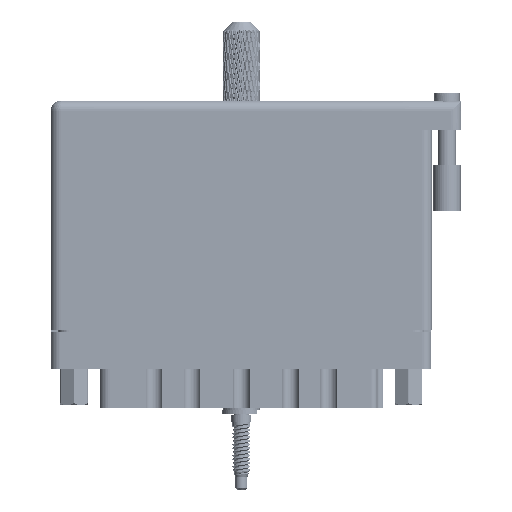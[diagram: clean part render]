
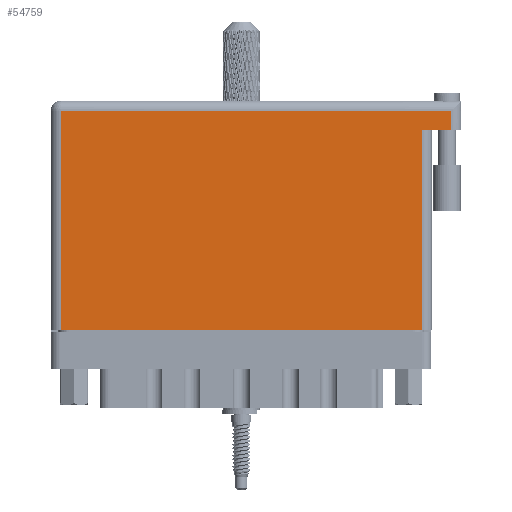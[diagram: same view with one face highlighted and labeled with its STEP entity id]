
A CAD part, front view. The second image highlights one B-rep face of the part: STEP entity #54759.
In plain terms, the highlighted face is planar.
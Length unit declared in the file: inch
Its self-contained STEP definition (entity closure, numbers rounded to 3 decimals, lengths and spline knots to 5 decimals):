
#682 = VERTEX_POINT ( 'NONE', #94941 ) ;
#1502 = VECTOR ( 'NONE', #6247, 39.37008 ) ;
#2481 = ORIENTED_EDGE ( 'NONE', *, *, #22006, .T. ) ;
#2527 = LINE ( 'NONE', #58421, #116686 ) ;
#3519 = EDGE_CURVE ( 'NONE', #682, #115316, #29239, .T. ) ;
#5059 = CARTESIAN_POINT ( 'NONE',  ( 0.07, 1.496, 0. ) ) ;
#6247 = DIRECTION ( 'NONE',  ( 1., 0., 0. ) ) ;
#7008 = ORIENTED_EDGE ( 'NONE', *, *, #46741, .T. ) ;
#7679 = VECTOR ( 'NONE', #100593, 39.37008 ) ;
#9228 = CARTESIAN_POINT ( 'NONE',  ( 2.8, 1.369, 0. ) ) ;
#10385 = VECTOR ( 'NONE', #109927, 39.37008 ) ;
#12273 = LINE ( 'NONE', #121031, #61718 ) ;
#16491 = VECTOR ( 'NONE', #57573, 39.37008 ) ;
#22006 = EDGE_CURVE ( 'NONE', #51543, #46863, #2527, .T. ) ;
#22716 = VERTEX_POINT ( 'NONE', #110933 ) ;
#28659 = CARTESIAN_POINT ( 'NONE',  ( 2.53, 1.369, 0. ) ) ;
#29239 = LINE ( 'NONE', #111358, #7679 ) ;
#31530 = CARTESIAN_POINT ( 'NONE',  ( 2.73, 1.566, 0. ) ) ;
#33336 = CARTESIAN_POINT ( 'NONE',  ( 0.07, 0., 0. ) ) ;
#33832 = EDGE_LOOP ( 'NONE', ( #79096, #118841, #110669, #79970, #2481, #7008 ) ) ;
#34595 = PLANE ( 'NONE',  #103821 ) ;
#35477 = DIRECTION ( 'NONE',  ( 0., 0., -1. ) ) ;
#39820 = EDGE_CURVE ( 'NONE', #22716, #115316, #98196, .T. ) ;
#41268 = EDGE_CURVE ( 'NONE', #22716, #51543, #49154, .T. ) ;
#46741 = EDGE_CURVE ( 'NONE', #46863, #60541, #12273, .T. ) ;
#46863 = VERTEX_POINT ( 'NONE', #5059 ) ;
#49154 = LINE ( 'NONE', #31530, #10385 ) ;
#51543 = VERTEX_POINT ( 'NONE', #127340 ) ;
#54759 = ADVANCED_FACE ( 'NONE', ( #103751 ), #34595, .F. ) ;
#55295 = DIRECTION ( 'NONE',  ( -1., 0., 0. ) ) ;
#57573 = DIRECTION ( 'NONE',  ( -1., 0., 0. ) ) ;
#58421 = CARTESIAN_POINT ( 'NONE',  ( 0., 1.496, 0. ) ) ;
#60541 = VERTEX_POINT ( 'NONE', #33336 ) ;
#61718 = VECTOR ( 'NONE', #121448, 39.37008 ) ;
#63704 = EDGE_CURVE ( 'NONE', #60541, #682, #124973, .T. ) ;
#64335 = CARTESIAN_POINT ( 'NONE',  ( 0., 1.566, 0. ) ) ;
#79096 = ORIENTED_EDGE ( 'NONE', *, *, #63704, .T. ) ;
#79970 = ORIENTED_EDGE ( 'NONE', *, *, #41268, .T. ) ;
#94941 = CARTESIAN_POINT ( 'NONE',  ( 2.53, 0., 0. ) ) ;
#98196 = LINE ( 'NONE', #9228, #16491 ) ;
#100593 = DIRECTION ( 'NONE',  ( 0., 1., 0. ) ) ;
#103751 = FACE_OUTER_BOUND ( 'NONE', #33832, .T. ) ;
#103821 = AXIS2_PLACEMENT_3D ( 'NONE', #64335, #35477, #55295 ) ;
#107051 = DIRECTION ( 'NONE',  ( -1., 0., 0. ) ) ;
#109927 = DIRECTION ( 'NONE',  ( 0., 1., 0. ) ) ;
#110669 = ORIENTED_EDGE ( 'NONE', *, *, #39820, .F. ) ;
#110933 = CARTESIAN_POINT ( 'NONE',  ( 2.73, 1.369, 0. ) ) ;
#111358 = CARTESIAN_POINT ( 'NONE',  ( 2.53, 1.369, 0. ) ) ;
#115316 = VERTEX_POINT ( 'NONE', #28659 ) ;
#116686 = VECTOR ( 'NONE', #107051, 39.37008 ) ;
#118841 = ORIENTED_EDGE ( 'NONE', *, *, #3519, .T. ) ;
#121031 = CARTESIAN_POINT ( 'NONE',  ( 0.07, 0., 0. ) ) ;
#121448 = DIRECTION ( 'NONE',  ( 0., -1., 0. ) ) ;
#124368 = CARTESIAN_POINT ( 'NONE',  ( 0., 0., 0. ) ) ;
#124973 = LINE ( 'NONE', #124368, #1502 ) ;
#127340 = CARTESIAN_POINT ( 'NONE',  ( 2.73, 1.496, 0. ) ) ;
